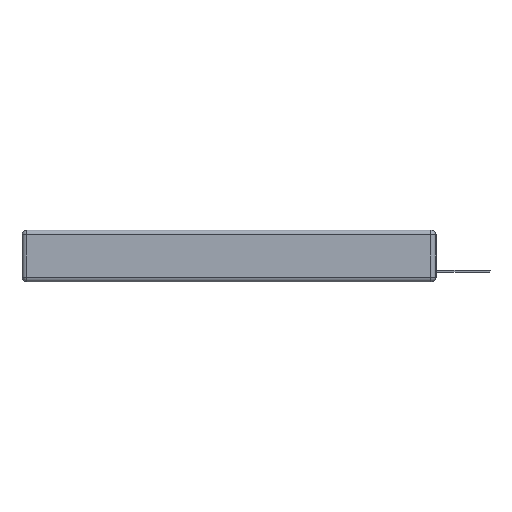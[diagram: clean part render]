
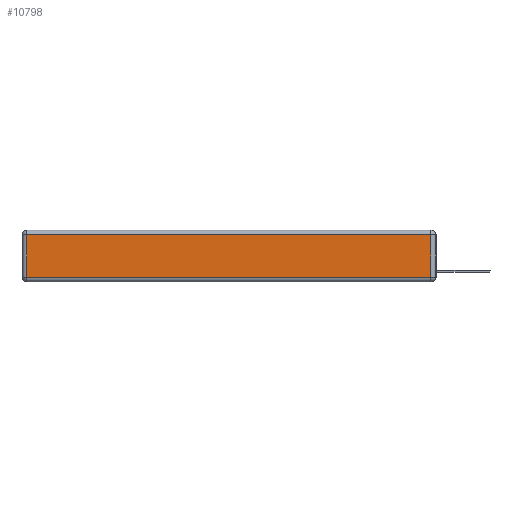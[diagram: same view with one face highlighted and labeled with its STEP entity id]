
A CAD part, left-side view. The second image highlights one B-rep face of the part: STEP entity #10798.
In plain terms, the highlighted planar face has unit normal (-1, 0, 0).
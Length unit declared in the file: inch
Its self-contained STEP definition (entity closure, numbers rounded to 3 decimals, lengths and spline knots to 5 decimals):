
#312 = LINE ( 'NONE', #5384, #5341 ) ;
#503 = DIRECTION ( 'NONE',  ( 0., 1., 0. ) ) ;
#807 = ORIENTED_EDGE ( 'NONE', *, *, #3525, .T. ) ;
#1090 = DIRECTION ( 'NONE',  ( 0., 0., -1. ) ) ;
#1364 = VERTEX_POINT ( 'NONE', #8577 ) ;
#1419 = VERTEX_POINT ( 'NONE', #3794 ) ;
#1491 = EDGE_LOOP ( 'NONE', ( #6707, #807, #8973, #7234 ) ) ;
#1679 = CARTESIAN_POINT ( 'NONE',  ( 0., 0.03, -0.343 ) ) ;
#1779 = LINE ( 'NONE', #11827, #6378 ) ;
#1981 = VERTEX_POINT ( 'NONE', #9925 ) ;
#2149 = DIRECTION ( 'NONE',  ( 0., -1., 0. ) ) ;
#2686 = PLANE ( 'NONE',  #9747 ) ;
#3248 = EDGE_CURVE ( 'NONE', #1364, #1419, #1779, .T. ) ;
#3525 = EDGE_CURVE ( 'NONE', #1981, #8360, #10797, .T. ) ;
#3794 = CARTESIAN_POINT ( 'NONE',  ( 0., 2.72, -0.313 ) ) ;
#4593 = DIRECTION ( 'NONE',  ( -1., 0., 0. ) ) ;
#5341 = VECTOR ( 'NONE', #503, 39.37008 ) ;
#5356 = EDGE_CURVE ( 'NONE', #1419, #1981, #7237, .T. ) ;
#5384 = CARTESIAN_POINT ( 'NONE',  ( 0., 2.75, -0.03 ) ) ;
#5705 = DIRECTION ( 'NONE',  ( 0., 0., 1. ) ) ;
#5920 = CARTESIAN_POINT ( 'NONE',  ( 0., 0.03, -0.03 ) ) ;
#6031 = CARTESIAN_POINT ( 'NONE',  ( 0., 0., -0.343 ) ) ;
#6378 = VECTOR ( 'NONE', #1090, 39.37008 ) ;
#6707 = ORIENTED_EDGE ( 'NONE', *, *, #5356, .T. ) ;
#7234 = ORIENTED_EDGE ( 'NONE', *, *, #3248, .T. ) ;
#7237 = LINE ( 'NONE', #8219, #10657 ) ;
#8219 = CARTESIAN_POINT ( 'NONE',  ( 0., 0., -0.313 ) ) ;
#8360 = VERTEX_POINT ( 'NONE', #5920 ) ;
#8577 = CARTESIAN_POINT ( 'NONE',  ( 0., 2.72, -0.03 ) ) ;
#8973 = ORIENTED_EDGE ( 'NONE', *, *, #12434, .T. ) ;
#9068 = DIRECTION ( 'NONE',  ( 0., 0., 1. ) ) ;
#9747 = AXIS2_PLACEMENT_3D ( 'NONE', #6031, #4593, #9068 ) ;
#9925 = CARTESIAN_POINT ( 'NONE',  ( 0., 0.03, -0.313 ) ) ;
#10657 = VECTOR ( 'NONE', #2149, 39.37008 ) ;
#10797 = LINE ( 'NONE', #1679, #11402 ) ;
#10798 = ADVANCED_FACE ( 'NONE', ( #10819 ), #2686, .T. ) ;
#10819 = FACE_OUTER_BOUND ( 'NONE', #1491, .T. ) ;
#11402 = VECTOR ( 'NONE', #5705, 39.37008 ) ;
#11827 = CARTESIAN_POINT ( 'NONE',  ( 0., 2.72, -0.343 ) ) ;
#12434 = EDGE_CURVE ( 'NONE', #8360, #1364, #312, .T. ) ;
